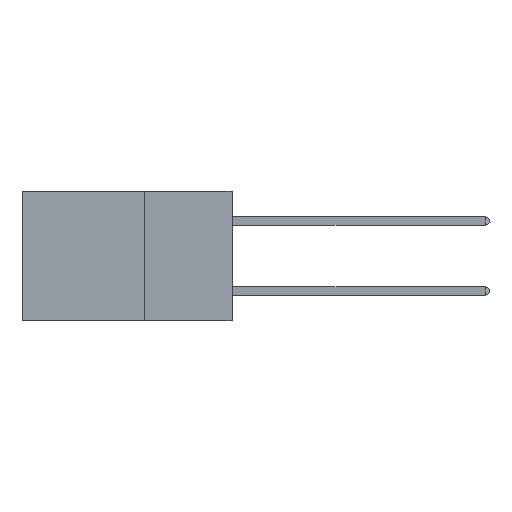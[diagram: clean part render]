
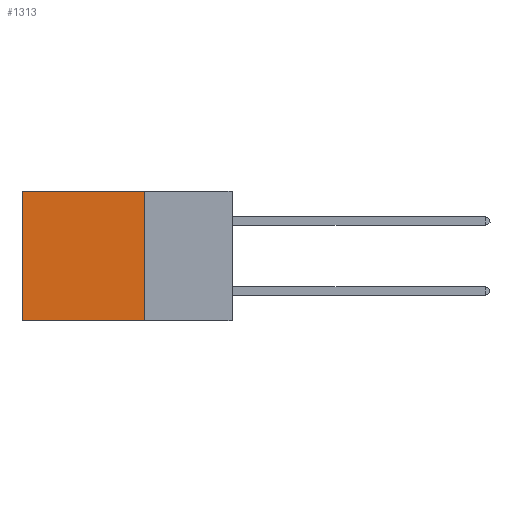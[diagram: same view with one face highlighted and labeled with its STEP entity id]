
A CAD part, left-side view. The second image highlights one B-rep face of the part: STEP entity #1313.
In plain terms, the highlighted planar face has unit normal (-1, 0, 0).
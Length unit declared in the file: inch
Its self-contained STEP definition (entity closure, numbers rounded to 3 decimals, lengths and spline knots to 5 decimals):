
#1138 = VECTOR ( 'NONE', #23630, 39.37008 ) ;
#1313 = ADVANCED_FACE ( 'NONE', ( #20442 ), #35561, .F. ) ;
#1609 = CARTESIAN_POINT ( 'NONE',  ( 0.2875, 0.25, -0.37 ) ) ;
#1620 = LINE ( 'NONE', #20708, #13721 ) ;
#4454 = DIRECTION ( 'NONE',  ( 0., 1., 0. ) ) ;
#4859 = VERTEX_POINT ( 'NONE', #6925 ) ;
#5128 = ORIENTED_EDGE ( 'NONE', *, *, #5220, .F. ) ;
#5220 = EDGE_CURVE ( 'NONE', #4859, #14605, #5874, .T. ) ;
#5617 = ORIENTED_EDGE ( 'NONE', *, *, #25710, .T. ) ;
#5874 = LINE ( 'NONE', #28802, #1138 ) ;
#6925 = CARTESIAN_POINT ( 'NONE',  ( 0.2875, 0.25, 0. ) ) ;
#7895 = CARTESIAN_POINT ( 'NONE',  ( 0.2875, 0.25, 0. ) ) ;
#11530 = EDGE_CURVE ( 'NONE', #14605, #35409, #32784, .T. ) ;
#11791 = CARTESIAN_POINT ( 'NONE',  ( 0.2875, 0.6, -0.37 ) ) ;
#11993 = AXIS2_PLACEMENT_3D ( 'NONE', #7895, #27500, #19285 ) ;
#12834 = CARTESIAN_POINT ( 'NONE',  ( 0.2875, 0.6, 0. ) ) ;
#13721 = VECTOR ( 'NONE', #4454, 39.37008 ) ;
#14605 = VERTEX_POINT ( 'NONE', #27126 ) ;
#17241 = ORIENTED_EDGE ( 'NONE', *, *, #17680, .T. ) ;
#17680 = EDGE_CURVE ( 'NONE', #4859, #27871, #1620, .T. ) ;
#19285 = DIRECTION ( 'NONE',  ( 0., 0., -1. ) ) ;
#20155 = LINE ( 'NONE', #26690, #32781 ) ;
#20442 = FACE_OUTER_BOUND ( 'NONE', #33077, .T. ) ;
#20708 = CARTESIAN_POINT ( 'NONE',  ( 0.2875, 0.25, 0. ) ) ;
#23630 = DIRECTION ( 'NONE',  ( 0., 0., -1. ) ) ;
#25710 = EDGE_CURVE ( 'NONE', #27871, #35409, #20155, .T. ) ;
#26134 = ORIENTED_EDGE ( 'NONE', *, *, #11530, .F. ) ;
#26690 = CARTESIAN_POINT ( 'NONE',  ( 0.2875, 0.6, 0. ) ) ;
#27126 = CARTESIAN_POINT ( 'NONE',  ( 0.2875, 0.25, -0.37 ) ) ;
#27500 = DIRECTION ( 'NONE',  ( 1., 0., 0. ) ) ;
#27871 = VERTEX_POINT ( 'NONE', #12834 ) ;
#28802 = CARTESIAN_POINT ( 'NONE',  ( 0.2875, 0.25, 0. ) ) ;
#30120 = VECTOR ( 'NONE', #35182, 39.37008 ) ;
#32411 = DIRECTION ( 'NONE',  ( 0., 0., -1. ) ) ;
#32781 = VECTOR ( 'NONE', #32411, 39.37008 ) ;
#32784 = LINE ( 'NONE', #1609, #30120 ) ;
#33077 = EDGE_LOOP ( 'NONE', ( #5617, #26134, #5128, #17241 ) ) ;
#35182 = DIRECTION ( 'NONE',  ( 0., 1., 0. ) ) ;
#35409 = VERTEX_POINT ( 'NONE', #11791 ) ;
#35561 = PLANE ( 'NONE',  #11993 ) ;
